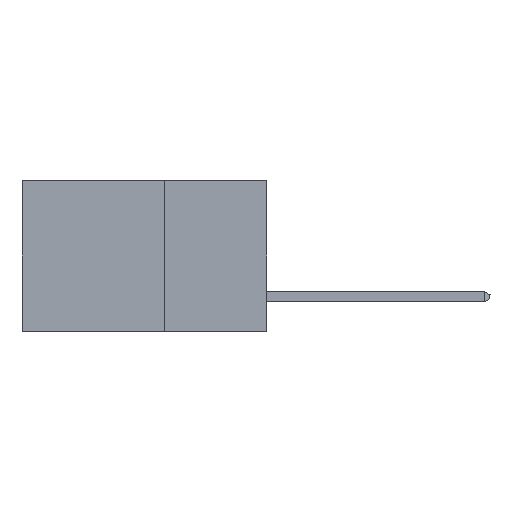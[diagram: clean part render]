
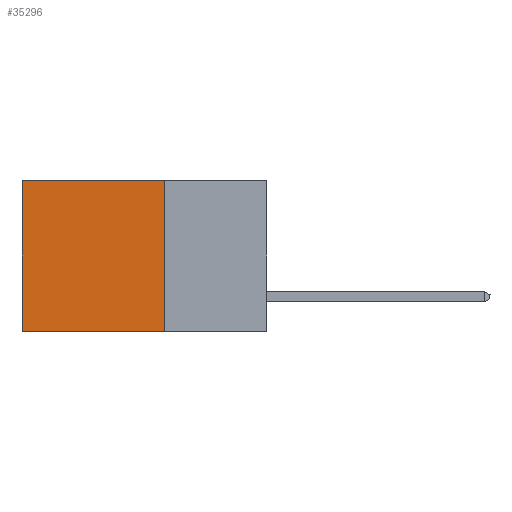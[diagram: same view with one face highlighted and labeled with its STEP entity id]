
A CAD part, left-side view. The second image highlights one B-rep face of the part: STEP entity #35296.
In plain terms, the highlighted planar face has unit normal (-1, 0, 0).
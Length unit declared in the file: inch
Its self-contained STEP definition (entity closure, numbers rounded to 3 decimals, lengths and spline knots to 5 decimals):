
#1164 = ORIENTED_EDGE ( 'NONE', *, *, #22088, .T. ) ;
#1168 = ORIENTED_EDGE ( 'NONE', *, *, #21784, .F. ) ;
#2295 = VECTOR ( 'NONE', #30634, 39.37008 ) ;
#3270 = CARTESIAN_POINT ( 'NONE',  ( 0.2875, 0.25, 0. ) ) ;
#3606 = LINE ( 'NONE', #28216, #23265 ) ;
#4734 = EDGE_CURVE ( 'NONE', #8342, #15879, #16872, .T. ) ;
#4803 = AXIS2_PLACEMENT_3D ( 'NONE', #3270, #22574, #20218 ) ;
#7835 = VERTEX_POINT ( 'NONE', #34484 ) ;
#8342 = VERTEX_POINT ( 'NONE', #27140 ) ;
#8656 = EDGE_LOOP ( 'NONE', ( #26857, #1168, #10199, #1164 ) ) ;
#9926 = DIRECTION ( 'NONE',  ( 0., 1., 0. ) ) ;
#10199 = ORIENTED_EDGE ( 'NONE', *, *, #35257, .F. ) ;
#13257 = CARTESIAN_POINT ( 'NONE',  ( 0.2875, 0.25, -0.37 ) ) ;
#14116 = DIRECTION ( 'NONE',  ( 0., 0., -1. ) ) ;
#15879 = VERTEX_POINT ( 'NONE', #25074 ) ;
#16872 = LINE ( 'NONE', #25196, #2295 ) ;
#18596 = CARTESIAN_POINT ( 'NONE',  ( 0.2875, 0.25, 0. ) ) ;
#18676 = CARTESIAN_POINT ( 'NONE',  ( 0.2875, 0.25, 0. ) ) ;
#20218 = DIRECTION ( 'NONE',  ( 0., 0., -1. ) ) ;
#21784 = EDGE_CURVE ( 'NONE', #7835, #15879, #22080, .T. ) ;
#22080 = LINE ( 'NONE', #13257, #30229 ) ;
#22088 = EDGE_CURVE ( 'NONE', #23858, #8342, #24205, .T. ) ;
#22574 = DIRECTION ( 'NONE',  ( 1., 0., 0. ) ) ;
#23265 = VECTOR ( 'NONE', #14116, 39.37008 ) ;
#23858 = VERTEX_POINT ( 'NONE', #18676 ) ;
#24205 = LINE ( 'NONE', #18596, #34295 ) ;
#25074 = CARTESIAN_POINT ( 'NONE',  ( 0.2875, 0.6, -0.37 ) ) ;
#25196 = CARTESIAN_POINT ( 'NONE',  ( 0.2875, 0.6, 0. ) ) ;
#25316 = PLANE ( 'NONE',  #4803 ) ;
#26857 = ORIENTED_EDGE ( 'NONE', *, *, #4734, .T. ) ;
#27140 = CARTESIAN_POINT ( 'NONE',  ( 0.2875, 0.6, 0. ) ) ;
#28044 = FACE_OUTER_BOUND ( 'NONE', #8656, .T. ) ;
#28216 = CARTESIAN_POINT ( 'NONE',  ( 0.2875, 0.25, 0. ) ) ;
#30229 = VECTOR ( 'NONE', #35532, 39.37008 ) ;
#30634 = DIRECTION ( 'NONE',  ( 0., 0., -1. ) ) ;
#34295 = VECTOR ( 'NONE', #9926, 39.37008 ) ;
#34484 = CARTESIAN_POINT ( 'NONE',  ( 0.2875, 0.25, -0.37 ) ) ;
#35257 = EDGE_CURVE ( 'NONE', #23858, #7835, #3606, .T. ) ;
#35296 = ADVANCED_FACE ( 'NONE', ( #28044 ), #25316, .F. ) ;
#35532 = DIRECTION ( 'NONE',  ( 0., 1., 0. ) ) ;
